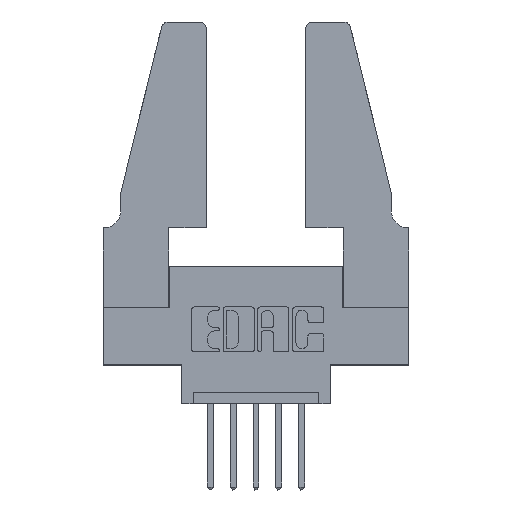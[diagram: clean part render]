
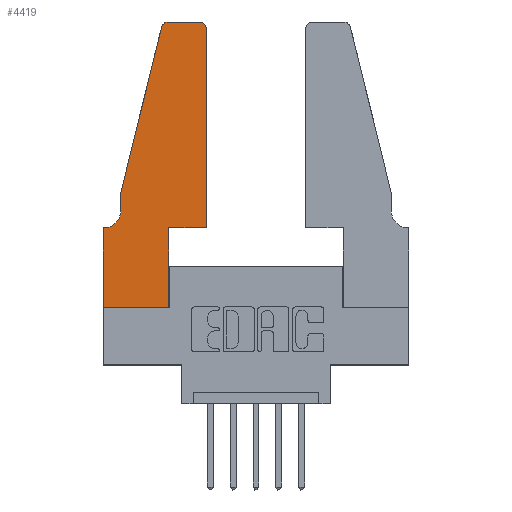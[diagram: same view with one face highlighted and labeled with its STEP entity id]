
A CAD part, top view. The second image highlights one B-rep face of the part: STEP entity #4419.
In plain terms, the highlighted planar face has unit normal (0, 0, 1).
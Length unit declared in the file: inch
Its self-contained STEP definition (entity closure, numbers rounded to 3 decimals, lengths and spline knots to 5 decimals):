
#108 = LINE ( 'NONE', #840, #1306 ) ;
#264 = CIRCLE ( 'NONE', #8644, 0.03 ) ;
#487 = ORIENTED_EDGE ( 'NONE', *, *, #8575, .T. ) ;
#840 = CARTESIAN_POINT ( 'NONE',  ( 0.4505, 0.35, 0.37 ) ) ;
#868 = VECTOR ( 'NONE', #8990, 39.37008 ) ;
#885 = CARTESIAN_POINT ( 'NONE',  ( 0.2865, 0.35, 0.37 ) ) ;
#974 = LINE ( 'NONE', #9279, #9806 ) ;
#1039 = EDGE_CURVE ( 'NONE', #7157, #7966, #974, .T. ) ;
#1044 = VECTOR ( 'NONE', #2945, 39.37008 ) ;
#1090 = CARTESIAN_POINT ( 'NONE',  ( 0.4205, 1.25, 0.37 ) ) ;
#1199 = VECTOR ( 'NONE', #1778, 39.37008 ) ;
#1306 = VECTOR ( 'NONE', #7619, 39.37008 ) ;
#1530 = VERTEX_POINT ( 'NONE', #1090 ) ;
#1602 = ORIENTED_EDGE ( 'NONE', *, *, #2671, .T. ) ;
#1778 = DIRECTION ( 'NONE',  ( 1., 0., 0. ) ) ;
#1788 = LINE ( 'NONE', #10029, #6336 ) ;
#1807 = DIRECTION ( 'NONE',  ( 1., 0., 0. ) ) ;
#1960 = DIRECTION ( 'NONE',  ( 1., 0., 0. ) ) ;
#1981 = CARTESIAN_POINT ( 'NONE',  ( 0.4505, 0.35, 0.37 ) ) ;
#2070 = DIRECTION ( 'NONE',  ( 0., 0., -1. ) ) ;
#2182 = DIRECTION ( 'NONE',  ( -1., 0., 0. ) ) ;
#2294 = DIRECTION ( 'NONE',  ( 0., -1., 0. ) ) ;
#2320 = EDGE_LOOP ( 'NONE', ( #10949, #6375, #5588, #3067, #8101, #7900, #7146, #1602, #487, #8329, #4497, #8680 ) ) ;
#2456 = EDGE_CURVE ( 'NONE', #3325, #3926, #264, .T. ) ;
#2610 = CARTESIAN_POINT ( 'NONE',  ( 0.284, 1.25, 0.37 ) ) ;
#2620 = EDGE_CURVE ( 'NONE', #3926, #7237, #5448, .T. ) ;
#2671 = EDGE_CURVE ( 'NONE', #7966, #6769, #3433, .T. ) ;
#2680 = LINE ( 'NONE', #3564, #8326 ) ;
#2752 = AXIS2_PLACEMENT_3D ( 'NONE', #5494, #2070, #6403 ) ;
#2782 = EDGE_CURVE ( 'NONE', #9420, #7687, #2680, .T. ) ;
#2785 = CARTESIAN_POINT ( 'NONE',  ( 0.4505, 1.22, 0.37 ) ) ;
#2868 = EDGE_CURVE ( 'NONE', #4713, #5002, #6586, .T. ) ;
#2884 = CARTESIAN_POINT ( 'NONE',  ( 0., 0., 0.37 ) ) ;
#2886 = CARTESIAN_POINT ( 'NONE',  ( 0.0755, 0.5, 0.37 ) ) ;
#2945 = DIRECTION ( 'NONE',  ( -1., 0., 0. ) ) ;
#3001 = CARTESIAN_POINT ( 'NONE',  ( 0., 0.35, 0.37 ) ) ;
#3067 = ORIENTED_EDGE ( 'NONE', *, *, #8241, .T. ) ;
#3325 = VERTEX_POINT ( 'NONE', #2610 ) ;
#3433 = LINE ( 'NONE', #10348, #1199 ) ;
#3564 = CARTESIAN_POINT ( 'NONE',  ( 0.4505, 0.35, 0.37 ) ) ;
#3921 = DIRECTION ( 'NONE',  ( 0., 0., 1. ) ) ;
#3923 = CARTESIAN_POINT ( 'NONE',  ( 0.0055, 0.35, 0.37 ) ) ;
#3926 = VERTEX_POINT ( 'NONE', #9560 ) ;
#4057 = LINE ( 'NONE', #9079, #9860 ) ;
#4419 = ADVANCED_FACE ( 'NONE', ( #6806 ), #4738, .T. ) ;
#4497 = ORIENTED_EDGE ( 'NONE', *, *, #5921, .T. ) ;
#4713 = VERTEX_POINT ( 'NONE', #8180 ) ;
#4738 = PLANE ( 'NONE',  #9551 ) ;
#4747 = CARTESIAN_POINT ( 'NONE',  ( 0.284, 1.22, 0.37 ) ) ;
#5002 = VERTEX_POINT ( 'NONE', #3923 ) ;
#5448 = LINE ( 'NONE', #7746, #8816 ) ;
#5485 = CARTESIAN_POINT ( 'NONE',  ( 0.0755, 0.35, 0.37 ) ) ;
#5494 = CARTESIAN_POINT ( 'NONE',  ( 0.0055, 0.42, 0.37 ) ) ;
#5588 = ORIENTED_EDGE ( 'NONE', *, *, #2620, .T. ) ;
#5854 = DIRECTION ( 'NONE',  ( 0., -1., 0. ) ) ;
#5921 = EDGE_CURVE ( 'NONE', #7687, #7659, #108, .T. ) ;
#5928 = DIRECTION ( 'NONE',  ( -0.239, -0.971, 0. ) ) ;
#6067 = DIRECTION ( 'NONE',  ( 0., 0., 1. ) ) ;
#6336 = VECTOR ( 'NONE', #2294, 39.37008 ) ;
#6375 = ORIENTED_EDGE ( 'NONE', *, *, #2456, .T. ) ;
#6403 = DIRECTION ( 'NONE',  ( -1., 0., 0. ) ) ;
#6447 = DIRECTION ( 'NONE',  ( 1., 0., 0. ) ) ;
#6502 = DIRECTION ( 'NONE',  ( 0., 0., 1. ) ) ;
#6586 = CIRCLE ( 'NONE', #2752, 0.07 ) ;
#6614 = EDGE_CURVE ( 'NONE', #5002, #7157, #10806, .T. ) ;
#6769 = VERTEX_POINT ( 'NONE', #8789 ) ;
#6806 = FACE_OUTER_BOUND ( 'NONE', #2320, .T. ) ;
#6948 = CARTESIAN_POINT ( 'NONE',  ( 0.4205, 1.22, 0.37 ) ) ;
#7146 = ORIENTED_EDGE ( 'NONE', *, *, #1039, .T. ) ;
#7157 = VERTEX_POINT ( 'NONE', #9590 ) ;
#7237 = VERTEX_POINT ( 'NONE', #2886 ) ;
#7527 = EDGE_CURVE ( 'NONE', #7659, #1530, #7678, .T. ) ;
#7566 = DIRECTION ( 'NONE',  ( 1., 0., 0. ) ) ;
#7619 = DIRECTION ( 'NONE',  ( 0., 1., 0. ) ) ;
#7659 = VERTEX_POINT ( 'NONE', #2785 ) ;
#7678 = CIRCLE ( 'NONE', #9720, 0.03 ) ;
#7687 = VERTEX_POINT ( 'NONE', #1981 ) ;
#7746 = CARTESIAN_POINT ( 'NONE',  ( 0.0755, 0.5, 0.37 ) ) ;
#7900 = ORIENTED_EDGE ( 'NONE', *, *, #6614, .T. ) ;
#7919 = LINE ( 'NONE', #8930, #868 ) ;
#7966 = VERTEX_POINT ( 'NONE', #2884 ) ;
#8101 = ORIENTED_EDGE ( 'NONE', *, *, #2868, .T. ) ;
#8180 = CARTESIAN_POINT ( 'NONE',  ( 0.0755, 0.42, 0.37 ) ) ;
#8241 = EDGE_CURVE ( 'NONE', #7237, #4713, #1788, .T. ) ;
#8326 = VECTOR ( 'NONE', #1960, 39.37008 ) ;
#8329 = ORIENTED_EDGE ( 'NONE', *, *, #2782, .T. ) ;
#8575 = EDGE_CURVE ( 'NONE', #6769, #9420, #7919, .T. ) ;
#8644 = AXIS2_PLACEMENT_3D ( 'NONE', #4747, #6502, #7566 ) ;
#8680 = ORIENTED_EDGE ( 'NONE', *, *, #7527, .T. ) ;
#8789 = CARTESIAN_POINT ( 'NONE',  ( 0.2865, 0., 0.37 ) ) ;
#8816 = VECTOR ( 'NONE', #5928, 39.37008 ) ;
#8930 = CARTESIAN_POINT ( 'NONE',  ( 0.2865, 0.35, 0.37 ) ) ;
#8990 = DIRECTION ( 'NONE',  ( 0., 1., 0. ) ) ;
#9079 = CARTESIAN_POINT ( 'NONE',  ( 0.2605, 1.25, 0.37 ) ) ;
#9279 = CARTESIAN_POINT ( 'NONE',  ( 0., 0., 0.37 ) ) ;
#9420 = VERTEX_POINT ( 'NONE', #885 ) ;
#9551 = AXIS2_PLACEMENT_3D ( 'NONE', #3001, #3921, #6447 ) ;
#9560 = CARTESIAN_POINT ( 'NONE',  ( 0.25487, 1.22718, 0.37 ) ) ;
#9590 = CARTESIAN_POINT ( 'NONE',  ( 0., 0.35, 0.37 ) ) ;
#9720 = AXIS2_PLACEMENT_3D ( 'NONE', #6948, #6067, #1807 ) ;
#9736 = EDGE_CURVE ( 'NONE', #1530, #3325, #4057, .T. ) ;
#9806 = VECTOR ( 'NONE', #5854, 39.37008 ) ;
#9860 = VECTOR ( 'NONE', #2182, 39.37008 ) ;
#10029 = CARTESIAN_POINT ( 'NONE',  ( 0.0755, 0.5, 0.37 ) ) ;
#10348 = CARTESIAN_POINT ( 'NONE',  ( 0., 0., 0.37 ) ) ;
#10806 = LINE ( 'NONE', #5485, #1044 ) ;
#10949 = ORIENTED_EDGE ( 'NONE', *, *, #9736, .T. ) ;
